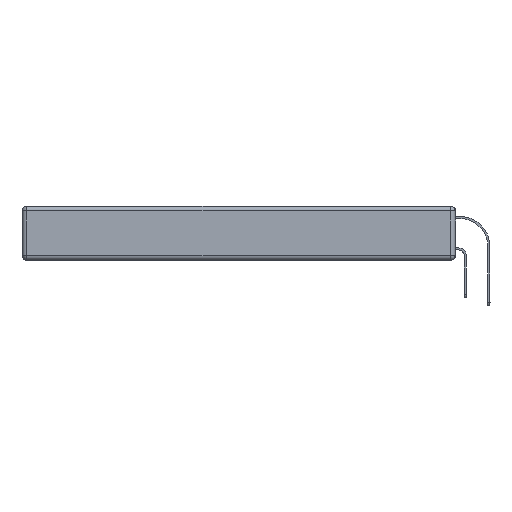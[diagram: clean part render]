
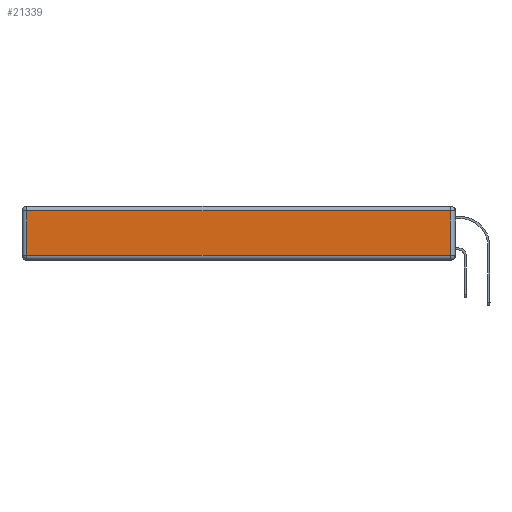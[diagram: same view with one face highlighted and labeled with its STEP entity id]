
A CAD part, left-side view. The second image highlights one B-rep face of the part: STEP entity #21339.
In plain terms, the highlighted planar face has unit normal (-1, 0, 0).
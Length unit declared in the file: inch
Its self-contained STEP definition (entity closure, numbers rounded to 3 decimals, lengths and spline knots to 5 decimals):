
#560 = ORIENTED_EDGE ( 'NONE', *, *, #1323, .T. ) ;
#791 = VECTOR ( 'NONE', #18670, 39.37008 ) ;
#1323 = EDGE_CURVE ( 'NONE', #11706, #7432, #6313, .T. ) ;
#2519 = DIRECTION ( 'NONE',  ( 0., 0., 1. ) ) ;
#4098 = EDGE_LOOP ( 'NONE', ( #8546, #16900, #560, #14774 ) ) ;
#4111 = LINE ( 'NONE', #5934, #6011 ) ;
#4306 = VERTEX_POINT ( 'NONE', #21039 ) ;
#5934 = CARTESIAN_POINT ( 'NONE',  ( 0., 0.03, -0.343 ) ) ;
#6011 = VECTOR ( 'NONE', #2519, 39.37008 ) ;
#6313 = LINE ( 'NONE', #13246, #791 ) ;
#6337 = AXIS2_PLACEMENT_3D ( 'NONE', #20640, #6686, #22345 ) ;
#6442 = LINE ( 'NONE', #20366, #11124 ) ;
#6478 = PLANE ( 'NONE',  #6337 ) ;
#6686 = DIRECTION ( 'NONE',  ( -1., 0., 0. ) ) ;
#6971 = CARTESIAN_POINT ( 'NONE',  ( 0., 0.03, -0.03 ) ) ;
#7432 = VERTEX_POINT ( 'NONE', #21878 ) ;
#7445 = CARTESIAN_POINT ( 'NONE',  ( 0., 2.72, -0.313 ) ) ;
#8546 = ORIENTED_EDGE ( 'NONE', *, *, #15281, .T. ) ;
#8763 = VECTOR ( 'NONE', #19053, 39.37008 ) ;
#10048 = CARTESIAN_POINT ( 'NONE',  ( 0., 0., -0.313 ) ) ;
#11124 = VECTOR ( 'NONE', #13799, 39.37008 ) ;
#11706 = VERTEX_POINT ( 'NONE', #6971 ) ;
#11853 = EDGE_CURVE ( 'NONE', #4306, #11706, #4111, .T. ) ;
#12823 = EDGE_CURVE ( 'NONE', #7432, #20137, #6442, .T. ) ;
#13246 = CARTESIAN_POINT ( 'NONE',  ( 0., 2.75, -0.03 ) ) ;
#13799 = DIRECTION ( 'NONE',  ( 0., 0., -1. ) ) ;
#14774 = ORIENTED_EDGE ( 'NONE', *, *, #12823, .T. ) ;
#15281 = EDGE_CURVE ( 'NONE', #20137, #4306, #15545, .T. ) ;
#15545 = LINE ( 'NONE', #10048, #8763 ) ;
#16900 = ORIENTED_EDGE ( 'NONE', *, *, #11853, .T. ) ;
#17237 = FACE_OUTER_BOUND ( 'NONE', #4098, .T. ) ;
#18670 = DIRECTION ( 'NONE',  ( 0., 1., 0. ) ) ;
#19053 = DIRECTION ( 'NONE',  ( 0., -1., 0. ) ) ;
#20137 = VERTEX_POINT ( 'NONE', #7445 ) ;
#20366 = CARTESIAN_POINT ( 'NONE',  ( 0., 2.72, -0.343 ) ) ;
#20640 = CARTESIAN_POINT ( 'NONE',  ( 0., 0., -0.343 ) ) ;
#21039 = CARTESIAN_POINT ( 'NONE',  ( 0., 0.03, -0.313 ) ) ;
#21339 = ADVANCED_FACE ( 'NONE', ( #17237 ), #6478, .T. ) ;
#21878 = CARTESIAN_POINT ( 'NONE',  ( 0., 2.72, -0.03 ) ) ;
#22345 = DIRECTION ( 'NONE',  ( 0., 0., 1. ) ) ;
